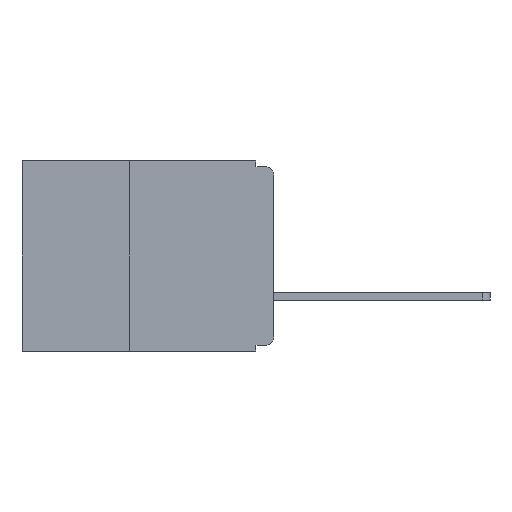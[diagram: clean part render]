
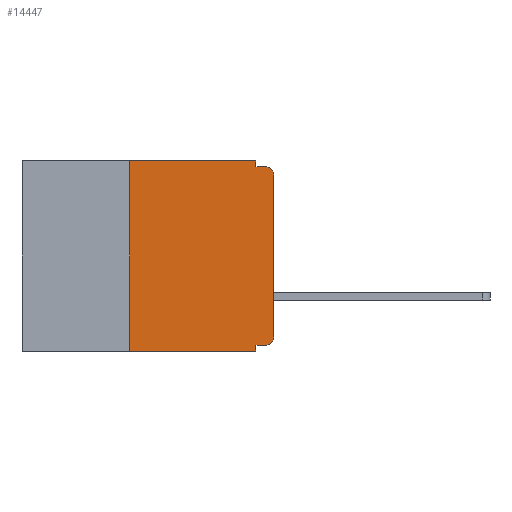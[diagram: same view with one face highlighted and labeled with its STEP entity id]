
A CAD part, left-side view. The second image highlights one B-rep face of the part: STEP entity #14447.
In plain terms, the highlighted planar face has unit normal (-1, 0, 0).
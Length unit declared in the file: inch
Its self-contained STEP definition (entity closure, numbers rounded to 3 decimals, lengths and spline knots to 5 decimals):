
#131 = LINE ( 'NONE', #5963, #23119 ) ;
#351 = ORIENTED_EDGE ( 'NONE', *, *, #20196, .T. ) ;
#640 = DIRECTION ( 'NONE',  ( 0., 0., -1. ) ) ;
#689 = LINE ( 'NONE', #8934, #7594 ) ;
#883 = EDGE_CURVE ( 'NONE', #4310, #13645, #11368, .T. ) ;
#1145 = ORIENTED_EDGE ( 'NONE', *, *, #25713, .T. ) ;
#1176 = ORIENTED_EDGE ( 'NONE', *, *, #20781, .F. ) ;
#1832 = CARTESIAN_POINT ( 'NONE',  ( 0., 0.25, 0. ) ) ;
#1903 = VECTOR ( 'NONE', #28675, 39.37008 ) ;
#2093 = DIRECTION ( 'NONE',  ( 0., 0., 1. ) ) ;
#2281 = LINE ( 'NONE', #6540, #25871 ) ;
#2539 = DIRECTION ( 'NONE',  ( 0., 1., 0. ) ) ;
#2719 = DIRECTION ( 'NONE',  ( -1., 0., 0. ) ) ;
#2770 = VERTEX_POINT ( 'NONE', #15746 ) ;
#3209 = EDGE_LOOP ( 'NONE', ( #351, #28633, #4052, #24064, #9094, #27951, #1145, #16296, #1176, #27308 ) ) ;
#3377 = LINE ( 'NONE', #26432, #1903 ) ;
#3469 = VERTEX_POINT ( 'NONE', #8342 ) ;
#4052 = ORIENTED_EDGE ( 'NONE', *, *, #27460, .F. ) ;
#4276 = DIRECTION ( 'NONE',  ( 0., 0., -1. ) ) ;
#4310 = VERTEX_POINT ( 'NONE', #1832 ) ;
#4748 = VECTOR ( 'NONE', #2539, 39.37008 ) ;
#4796 = CIRCLE ( 'NONE', #24382, 0.015 ) ;
#4945 = VERTEX_POINT ( 'NONE', #27313 ) ;
#5661 = AXIS2_PLACEMENT_3D ( 'NONE', #15722, #18057, #4276 ) ;
#5963 = CARTESIAN_POINT ( 'NONE',  ( 0., 0.031, -0.33 ) ) ;
#6540 = CARTESIAN_POINT ( 'NONE',  ( 0., 0., 0. ) ) ;
#7434 = CARTESIAN_POINT ( 'NONE',  ( 0., 0.437, 0. ) ) ;
#7594 = VECTOR ( 'NONE', #2093, 39.37008 ) ;
#8342 = CARTESIAN_POINT ( 'NONE',  ( 0., 0.015, -0.32 ) ) ;
#8934 = CARTESIAN_POINT ( 'NONE',  ( 0., 0.25, -0.33 ) ) ;
#9094 = ORIENTED_EDGE ( 'NONE', *, *, #883, .F. ) ;
#9508 = EDGE_CURVE ( 'NONE', #14677, #10008, #131, .T. ) ;
#9682 = CARTESIAN_POINT ( 'NONE',  ( 0., 0.031, -0.32 ) ) ;
#9832 = CIRCLE ( 'NONE', #11715, 0.015 ) ;
#9866 = CARTESIAN_POINT ( 'NONE',  ( 0., 0., -0.025 ) ) ;
#10008 = VERTEX_POINT ( 'NONE', #26496 ) ;
#10397 = EDGE_CURVE ( 'NONE', #3469, #16944, #4796, .T. ) ;
#10486 = DIRECTION ( 'NONE',  ( 0., 0., -1. ) ) ;
#10528 = CARTESIAN_POINT ( 'NONE',  ( 0., 0., -0.01 ) ) ;
#11368 = LINE ( 'NONE', #7434, #16793 ) ;
#11715 = AXIS2_PLACEMENT_3D ( 'NONE', #16503, #2719, #18790 ) ;
#13383 = CARTESIAN_POINT ( 'NONE',  ( 0., 0.437, -0.33 ) ) ;
#13645 = VERTEX_POINT ( 'NONE', #19838 ) ;
#13798 = VECTOR ( 'NONE', #28712, 39.37008 ) ;
#13972 = CARTESIAN_POINT ( 'NONE',  ( 0., 0., -0.32 ) ) ;
#14447 = ADVANCED_FACE ( 'NONE', ( #17226 ), #29272, .F. ) ;
#14469 = DIRECTION ( 'NONE',  ( -1., 0., 0. ) ) ;
#14677 = VERTEX_POINT ( 'NONE', #9682 ) ;
#15722 = CARTESIAN_POINT ( 'NONE',  ( 0., 0.437, 0. ) ) ;
#15726 = DIRECTION ( 'NONE',  ( 0., -1., 0. ) ) ;
#15746 = CARTESIAN_POINT ( 'NONE',  ( 0., 0.031, -0.01 ) ) ;
#16296 = ORIENTED_EDGE ( 'NONE', *, *, #9508, .F. ) ;
#16503 = CARTESIAN_POINT ( 'NONE',  ( 0., 0.015, -0.025 ) ) ;
#16793 = VECTOR ( 'NONE', #23705, 39.37008 ) ;
#16944 = VERTEX_POINT ( 'NONE', #19422 ) ;
#17002 = LINE ( 'NONE', #13972, #4748 ) ;
#17062 = VERTEX_POINT ( 'NONE', #19891 ) ;
#17226 = FACE_OUTER_BOUND ( 'NONE', #3209, .T. ) ;
#17865 = EDGE_CURVE ( 'NONE', #28499, #17062, #9832, .T. ) ;
#18057 = DIRECTION ( 'NONE',  ( 1., 0., 0. ) ) ;
#18790 = DIRECTION ( 'NONE',  ( 0., 0., -1. ) ) ;
#19422 = CARTESIAN_POINT ( 'NONE',  ( 0., 0., -0.305 ) ) ;
#19838 = CARTESIAN_POINT ( 'NONE',  ( 0., 0.031, 0. ) ) ;
#19891 = CARTESIAN_POINT ( 'NONE',  ( 0., 0.015, -0.01 ) ) ;
#20196 = EDGE_CURVE ( 'NONE', #16944, #28499, #2281, .T. ) ;
#20781 = EDGE_CURVE ( 'NONE', #3469, #14677, #17002, .T. ) ;
#23119 = VECTOR ( 'NONE', #10486, 39.37008 ) ;
#23451 = LINE ( 'NONE', #13383, #28720 ) ;
#23705 = DIRECTION ( 'NONE',  ( 0., -1., 0. ) ) ;
#24064 = ORIENTED_EDGE ( 'NONE', *, *, #28078, .F. ) ;
#24382 = AXIS2_PLACEMENT_3D ( 'NONE', #28050, #14469, #640 ) ;
#24786 = DIRECTION ( 'NONE',  ( 0., 0., 1. ) ) ;
#25713 = EDGE_CURVE ( 'NONE', #4945, #10008, #23451, .T. ) ;
#25871 = VECTOR ( 'NONE', #24786, 39.37008 ) ;
#25918 = LINE ( 'NONE', #10528, #13798 ) ;
#26432 = CARTESIAN_POINT ( 'NONE',  ( 0., 0.031, 0. ) ) ;
#26496 = CARTESIAN_POINT ( 'NONE',  ( 0., 0.031, -0.33 ) ) ;
#27308 = ORIENTED_EDGE ( 'NONE', *, *, #10397, .T. ) ;
#27313 = CARTESIAN_POINT ( 'NONE',  ( 0., 0.25, -0.33 ) ) ;
#27460 = EDGE_CURVE ( 'NONE', #2770, #17062, #25918, .T. ) ;
#27951 = ORIENTED_EDGE ( 'NONE', *, *, #29619, .F. ) ;
#28050 = CARTESIAN_POINT ( 'NONE',  ( 0., 0.015, -0.305 ) ) ;
#28078 = EDGE_CURVE ( 'NONE', #13645, #2770, #3377, .T. ) ;
#28499 = VERTEX_POINT ( 'NONE', #9866 ) ;
#28633 = ORIENTED_EDGE ( 'NONE', *, *, #17865, .T. ) ;
#28675 = DIRECTION ( 'NONE',  ( 0., 0., -1. ) ) ;
#28712 = DIRECTION ( 'NONE',  ( 0., -1., 0. ) ) ;
#28720 = VECTOR ( 'NONE', #15726, 39.37008 ) ;
#29272 = PLANE ( 'NONE',  #5661 ) ;
#29619 = EDGE_CURVE ( 'NONE', #4945, #4310, #689, .T. ) ;
